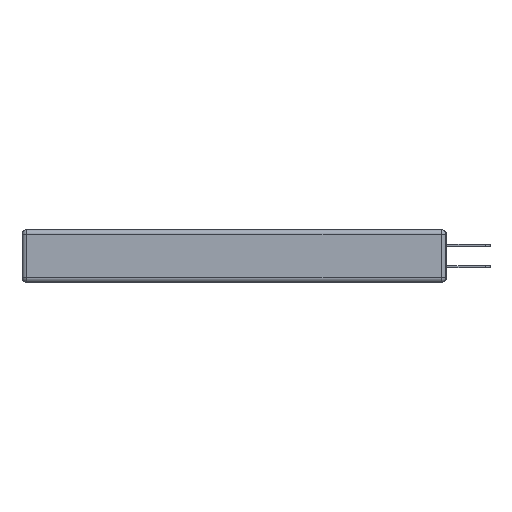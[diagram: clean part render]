
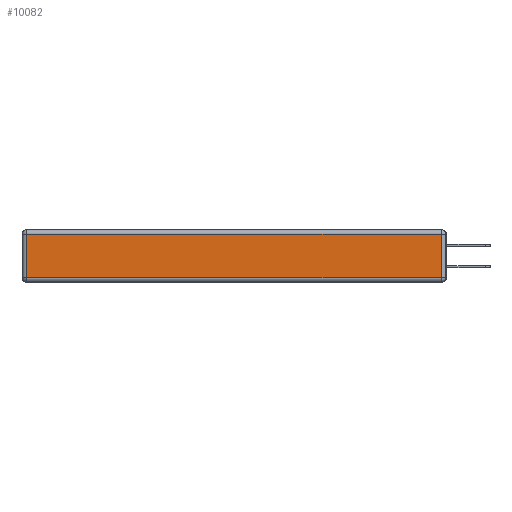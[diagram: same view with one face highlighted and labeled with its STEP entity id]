
A CAD part, left-side view. The second image highlights one B-rep face of the part: STEP entity #10082.
In plain terms, the highlighted planar face has unit normal (-1, 0, 0).
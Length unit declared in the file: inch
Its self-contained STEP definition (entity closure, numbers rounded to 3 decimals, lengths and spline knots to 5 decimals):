
#827 = LINE ( 'NONE', #16685, #19534 ) ;
#1018 = LINE ( 'NONE', #25171, #15621 ) ;
#1186 = EDGE_CURVE ( 'NONE', #5060, #26077, #20592, .T. ) ;
#2011 = ORIENTED_EDGE ( 'NONE', *, *, #24328, .T. ) ;
#2574 = EDGE_LOOP ( 'NONE', ( #5336, #9605, #21713, #2011 ) ) ;
#3884 = CARTESIAN_POINT ( 'NONE',  ( 0., 0., -0.313 ) ) ;
#4118 = VERTEX_POINT ( 'NONE', #12163 ) ;
#5060 = VERTEX_POINT ( 'NONE', #25897 ) ;
#5209 = PLANE ( 'NONE',  #15779 ) ;
#5336 = ORIENTED_EDGE ( 'NONE', *, *, #1186, .T. ) ;
#6031 = DIRECTION ( 'NONE',  ( 0., -1., 0. ) ) ;
#9068 = VERTEX_POINT ( 'NONE', #15608 ) ;
#9583 = VECTOR ( 'NONE', #12135, 39.37008 ) ;
#9605 = ORIENTED_EDGE ( 'NONE', *, *, #15187, .T. ) ;
#10082 = ADVANCED_FACE ( 'NONE', ( #22815 ), #5209, .T. ) ;
#12135 = DIRECTION ( 'NONE',  ( 0., 0., 1. ) ) ;
#12163 = CARTESIAN_POINT ( 'NONE',  ( 0., 0.03, -0.03 ) ) ;
#12489 = DIRECTION ( 'NONE',  ( 0., 0., 1. ) ) ;
#12761 = CARTESIAN_POINT ( 'NONE',  ( 0., 0.03, -0.313 ) ) ;
#14172 = DIRECTION ( 'NONE',  ( 0., 1., 0. ) ) ;
#14712 = CARTESIAN_POINT ( 'NONE',  ( 0., 0., -0.343 ) ) ;
#15065 = LINE ( 'NONE', #16367, #9583 ) ;
#15187 = EDGE_CURVE ( 'NONE', #26077, #4118, #15065, .T. ) ;
#15608 = CARTESIAN_POINT ( 'NONE',  ( 0., 2.72, -0.03 ) ) ;
#15621 = VECTOR ( 'NONE', #14172, 39.37008 ) ;
#15779 = AXIS2_PLACEMENT_3D ( 'NONE', #14712, #27881, #12489 ) ;
#16367 = CARTESIAN_POINT ( 'NONE',  ( 0., 0.03, -0.343 ) ) ;
#16685 = CARTESIAN_POINT ( 'NONE',  ( 0., 2.72, -0.343 ) ) ;
#19534 = VECTOR ( 'NONE', #20942, 39.37008 ) ;
#20592 = LINE ( 'NONE', #3884, #25665 ) ;
#20942 = DIRECTION ( 'NONE',  ( 0., 0., -1. ) ) ;
#21713 = ORIENTED_EDGE ( 'NONE', *, *, #27662, .T. ) ;
#22815 = FACE_OUTER_BOUND ( 'NONE', #2574, .T. ) ;
#24328 = EDGE_CURVE ( 'NONE', #9068, #5060, #827, .T. ) ;
#25171 = CARTESIAN_POINT ( 'NONE',  ( 0., 2.75, -0.03 ) ) ;
#25665 = VECTOR ( 'NONE', #6031, 39.37008 ) ;
#25897 = CARTESIAN_POINT ( 'NONE',  ( 0., 2.72, -0.313 ) ) ;
#26077 = VERTEX_POINT ( 'NONE', #12761 ) ;
#27662 = EDGE_CURVE ( 'NONE', #4118, #9068, #1018, .T. ) ;
#27881 = DIRECTION ( 'NONE',  ( -1., 0., 0. ) ) ;
